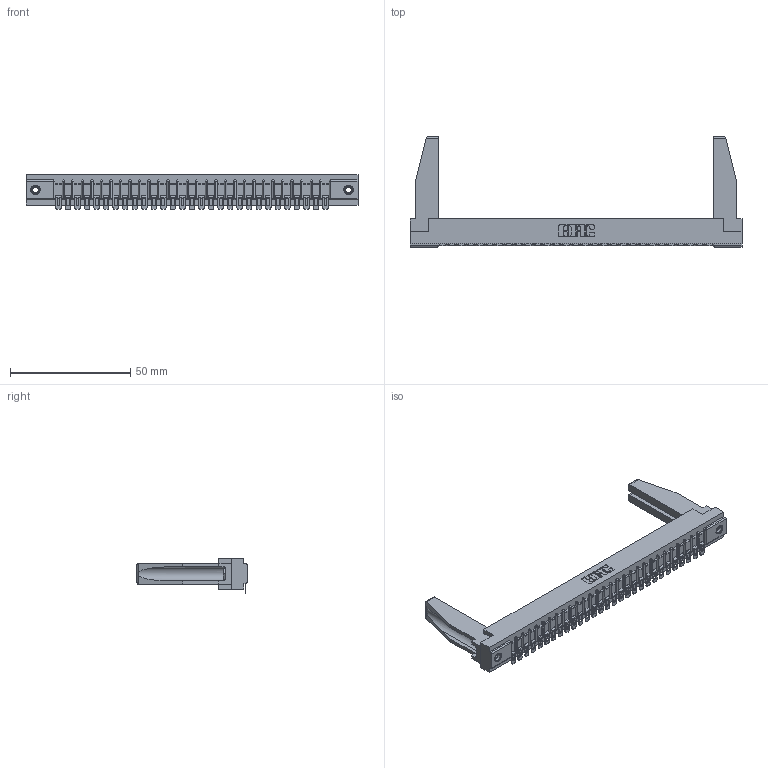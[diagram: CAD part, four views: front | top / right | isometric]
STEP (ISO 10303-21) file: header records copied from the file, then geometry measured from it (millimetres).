
FILE_DESCRIPTION (( 'STEP AP203' ), '1' );
FILE_NAME ('307-029-554-178.STEP', '2019-09-05T03:53:19', ( '' ), ( '' ), 'SwSTEP 2.0', 'SolidWorks 2016', '' );
FILE_SCHEMA (( 'CONFIG_CONTROL_DESIGN' ));
Length unit declared in the file: inch
Products named in the file (5): 345-250-001_345-250-001-102; 307 Part_.156 Dia Mounting Holes; 307-029-554-178; 307-290-002_554; 307-220-078
Assembly tree (34 placements, depth 2):
  307-029-554-178
    307 Part_.156 Dia Mounting Holes
    307-290-002_554  x29
    307-220-078  x2
    345-250-001_345-250-001-102  x2
Bounding box: 137.92 x 45.72 x 14.52 mm (x, y, z)
Volume: 18666.2 mm3; surface area: 22101.6 mm2
Topology: 34 solids, 34 shells, 2627 faces, 7990 edges, 5236 vertices
Faces by surface type: plane 1488, cylinder 1063, sphere 60, cone 12, torus 4
Entity records: 29868 total; most frequent: CARTESIAN_POINT 5036, ORIENTED_EDGE 4982, DIRECTION 4861, EDGE_CURVE 2491, VECTOR 1899, LINE 1899, VERTEX_POINT 1614, AXIS2_PLACEMENT_3D 1481
